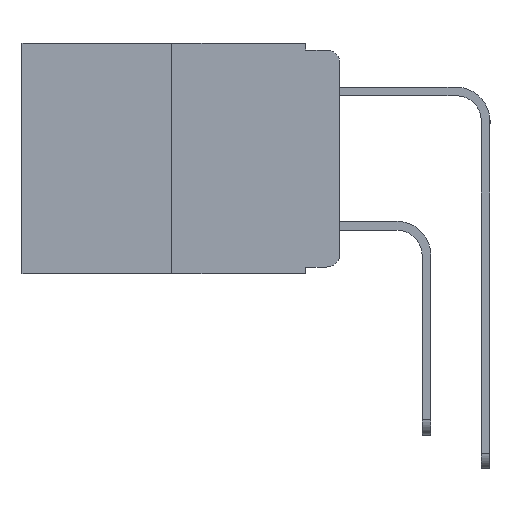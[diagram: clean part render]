
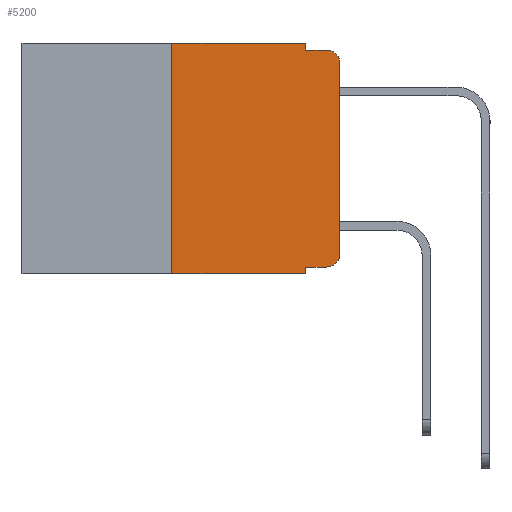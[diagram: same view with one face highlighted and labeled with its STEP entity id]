
A CAD part, left-side view. The second image highlights one B-rep face of the part: STEP entity #5200.
In plain terms, the highlighted planar face has unit normal (-1, 0, 0).
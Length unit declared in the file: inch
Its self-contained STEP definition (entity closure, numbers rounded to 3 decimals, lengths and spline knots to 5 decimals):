
#386 = AXIS2_PLACEMENT_3D ( 'NONE', #14564, #6389, #15937 ) ;
#441 = AXIS2_PLACEMENT_3D ( 'NONE', #7543, #17046, #8896 ) ;
#471 = CARTESIAN_POINT ( 'NONE',  ( 0., 0.051, 0. ) ) ;
#627 = ORIENTED_EDGE ( 'NONE', *, *, #8799, .F. ) ;
#936 = CARTESIAN_POINT ( 'NONE',  ( 0., 0.25, 0. ) ) ;
#1111 = VERTEX_POINT ( 'NONE', #5880 ) ;
#1740 = CARTESIAN_POINT ( 'NONE',  ( 0., 0.051, -0.01 ) ) ;
#1838 = ORIENTED_EDGE ( 'NONE', *, *, #7315, .F. ) ;
#1931 = VERTEX_POINT ( 'NONE', #14148 ) ;
#1945 = CARTESIAN_POINT ( 'NONE',  ( 0., 0.051, -0.333 ) ) ;
#2008 = DIRECTION ( 'NONE',  ( 0., -1., 0. ) ) ;
#2287 = VERTEX_POINT ( 'NONE', #9773 ) ;
#2339 = VECTOR ( 'NONE', #16577, 39.37008 ) ;
#2378 = LINE ( 'NONE', #11583, #9411 ) ;
#2390 = VERTEX_POINT ( 'NONE', #13605 ) ;
#3308 = DIRECTION ( 'NONE',  ( 0., -1., 0. ) ) ;
#3763 = VERTEX_POINT ( 'NONE', #471 ) ;
#3833 = AXIS2_PLACEMENT_3D ( 'NONE', #5191, #5790, #5770 ) ;
#4470 = CIRCLE ( 'NONE', #386, 0.02 ) ;
#4913 = LINE ( 'NONE', #1945, #14969 ) ;
#4936 = CARTESIAN_POINT ( 'NONE',  ( 0., 0.25, 0. ) ) ;
#5025 = VERTEX_POINT ( 'NONE', #7373 ) ;
#5089 = VECTOR ( 'NONE', #6377, 39.37008 ) ;
#5191 = CARTESIAN_POINT ( 'NONE',  ( 0., 0.473, 0. ) ) ;
#5200 = ADVANCED_FACE ( 'NONE', ( #9636 ), #5809, .F. ) ;
#5544 = LINE ( 'NONE', #6824, #5089 ) ;
#5770 = DIRECTION ( 'NONE',  ( 0., 0., -1. ) ) ;
#5790 = DIRECTION ( 'NONE',  ( 1., 0., 0. ) ) ;
#5804 = LINE ( 'NONE', #1740, #16250 ) ;
#5809 = PLANE ( 'NONE',  #3833 ) ;
#5880 = CARTESIAN_POINT ( 'NONE',  ( 0., 0.25, -0.343 ) ) ;
#6124 = VERTEX_POINT ( 'NONE', #8626 ) ;
#6377 = DIRECTION ( 'NONE',  ( 0., -1., 0. ) ) ;
#6389 = DIRECTION ( 'NONE',  ( -1., 0., 0. ) ) ;
#6824 = CARTESIAN_POINT ( 'NONE',  ( 0., 0.473, -0.343 ) ) ;
#7315 = EDGE_CURVE ( 'NONE', #9490, #3763, #13439, .T. ) ;
#7373 = CARTESIAN_POINT ( 'NONE',  ( 0., 0.051, -0.343 ) ) ;
#7523 = EDGE_CURVE ( 'NONE', #1111, #5025, #5544, .T. ) ;
#7543 = CARTESIAN_POINT ( 'NONE',  ( 0., 0.02, -0.03 ) ) ;
#8149 = LINE ( 'NONE', #15873, #12217 ) ;
#8550 = LINE ( 'NONE', #4936, #15386 ) ;
#8626 = CARTESIAN_POINT ( 'NONE',  ( 0., 0.02, -0.01 ) ) ;
#8745 = EDGE_CURVE ( 'NONE', #2287, #2390, #2378, .T. ) ;
#8748 = EDGE_CURVE ( 'NONE', #2390, #6124, #9836, .T. ) ;
#8750 = EDGE_CURVE ( 'NONE', #8771, #6124, #5804, .T. ) ;
#8771 = VERTEX_POINT ( 'NONE', #14390 ) ;
#8796 = EDGE_CURVE ( 'NONE', #3763, #8771, #8986, .T. ) ;
#8799 = EDGE_CURVE ( 'NONE', #1111, #9490, #8550, .T. ) ;
#8801 = EDGE_CURVE ( 'NONE', #15640, #5025, #8149, .T. ) ;
#8820 = EDGE_CURVE ( 'NONE', #15640, #1931, #4913, .T. ) ;
#8825 = EDGE_CURVE ( 'NONE', #1931, #2287, #4470, .T. ) ;
#8896 = DIRECTION ( 'NONE',  ( 0., 0., -1. ) ) ;
#8954 = DIRECTION ( 'NONE',  ( 0., 0., -1. ) ) ;
#8986 = LINE ( 'NONE', #9012, #11772 ) ;
#9012 = CARTESIAN_POINT ( 'NONE',  ( 0., 0.051, 0. ) ) ;
#9411 = VECTOR ( 'NONE', #12973, 39.37008 ) ;
#9490 = VERTEX_POINT ( 'NONE', #936 ) ;
#9636 = FACE_OUTER_BOUND ( 'NONE', #10054, .T. ) ;
#9773 = CARTESIAN_POINT ( 'NONE',  ( 0., 0., -0.313 ) ) ;
#9836 = CIRCLE ( 'NONE', #441, 0.02 ) ;
#10054 = EDGE_LOOP ( 'NONE', ( #12027, #16623, #11486, #14752, #1838, #627, #17225, #10833, #11268, #14447 ) ) ;
#10833 = ORIENTED_EDGE ( 'NONE', *, *, #8801, .F. ) ;
#11268 = ORIENTED_EDGE ( 'NONE', *, *, #8820, .T. ) ;
#11486 = ORIENTED_EDGE ( 'NONE', *, *, #8750, .F. ) ;
#11583 = CARTESIAN_POINT ( 'NONE',  ( 0., 0., 0. ) ) ;
#11772 = VECTOR ( 'NONE', #8954, 39.37008 ) ;
#12027 = ORIENTED_EDGE ( 'NONE', *, *, #8745, .T. ) ;
#12217 = VECTOR ( 'NONE', #17220, 39.37008 ) ;
#12973 = DIRECTION ( 'NONE',  ( 0., 0., 1. ) ) ;
#13144 = DIRECTION ( 'NONE',  ( 0., 0., 1. ) ) ;
#13439 = LINE ( 'NONE', #15603, #2339 ) ;
#13605 = CARTESIAN_POINT ( 'NONE',  ( 0., 0., -0.03 ) ) ;
#14148 = CARTESIAN_POINT ( 'NONE',  ( 0., 0.02, -0.333 ) ) ;
#14390 = CARTESIAN_POINT ( 'NONE',  ( 0., 0.051, -0.01 ) ) ;
#14447 = ORIENTED_EDGE ( 'NONE', *, *, #8825, .T. ) ;
#14564 = CARTESIAN_POINT ( 'NONE',  ( 0., 0.02, -0.313 ) ) ;
#14752 = ORIENTED_EDGE ( 'NONE', *, *, #8796, .F. ) ;
#14969 = VECTOR ( 'NONE', #2008, 39.37008 ) ;
#15386 = VECTOR ( 'NONE', #13144, 39.37008 ) ;
#15603 = CARTESIAN_POINT ( 'NONE',  ( 0., 0.473, 0. ) ) ;
#15640 = VERTEX_POINT ( 'NONE', #15711 ) ;
#15711 = CARTESIAN_POINT ( 'NONE',  ( 0., 0.051, -0.333 ) ) ;
#15873 = CARTESIAN_POINT ( 'NONE',  ( 0., 0.051, 0. ) ) ;
#15937 = DIRECTION ( 'NONE',  ( 0., 0., -1. ) ) ;
#16250 = VECTOR ( 'NONE', #3308, 39.37008 ) ;
#16577 = DIRECTION ( 'NONE',  ( 0., -1., 0. ) ) ;
#16623 = ORIENTED_EDGE ( 'NONE', *, *, #8748, .T. ) ;
#17046 = DIRECTION ( 'NONE',  ( -1., 0., 0. ) ) ;
#17220 = DIRECTION ( 'NONE',  ( 0., 0., -1. ) ) ;
#17225 = ORIENTED_EDGE ( 'NONE', *, *, #7523, .T. ) ;
